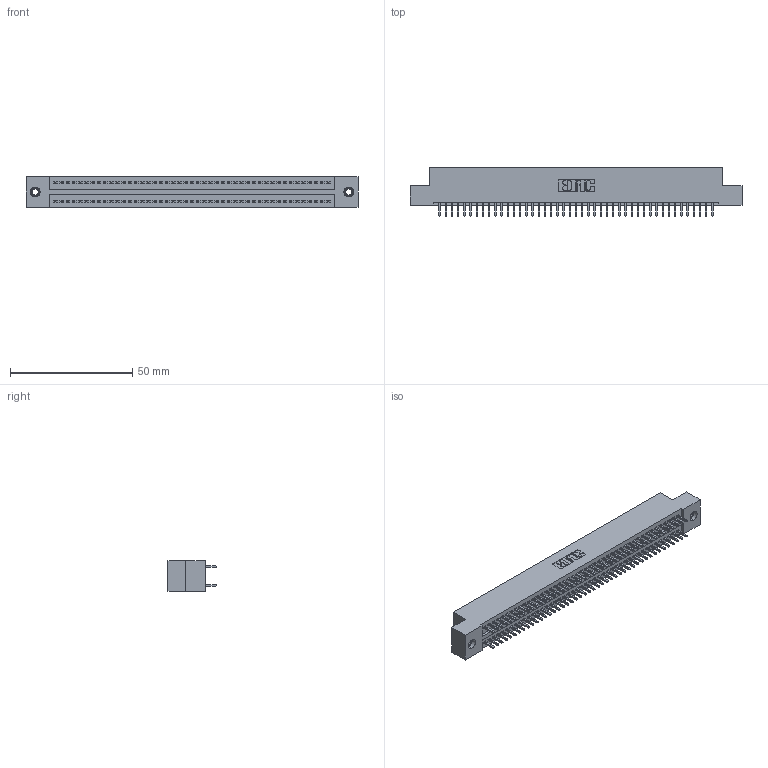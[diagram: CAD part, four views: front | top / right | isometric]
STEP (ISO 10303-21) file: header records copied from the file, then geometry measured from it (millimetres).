
FILE_DESCRIPTION (( 'STEP AP203' ), '1' );
FILE_NAME ('325-090-520-207.STEP', '2020-02-25T05:37:34', ( '' ), ( '' ), 'SwSTEP 2.0', 'SolidWorks 2016', '' );
FILE_SCHEMA (( 'CONFIG_CONTROL_DESIGN' ));
Length unit declared in the file: inch
Products named in the file (4): 325-090-520-207; 325 Part_TI; 345-250-001_345-250-005-103; 325-292-001_325-293-120
Assembly tree (93 placements, depth 2):
  325-090-520-207
    325 Part_TI
    325-292-001_325-293-120  x90
    345-250-001_345-250-005-103  x2
Bounding box: 136.02 x 19.68 x 12.45 mm (x, y, z)
Volume: 17559.1 mm3; surface area: 21168.5 mm2
Topology: 93 solids, 93 shells, 4854 faces, 14397 edges, 9470 vertices
Faces by surface type: plane 3342, cylinder 1496, cone 12, torus 4
Entity records: 29766 total; most frequent: CARTESIAN_POINT 4913, ORIENTED_EDGE 4842, DIRECTION 4223, EDGE_CURVE 2421, LINE 2273, VECTOR 2273, VERTEX_POINT 1608, AXIS2_PLACEMENT_3D 975
